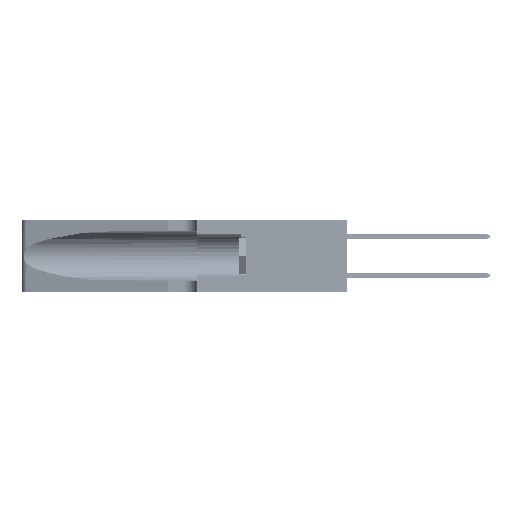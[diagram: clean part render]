
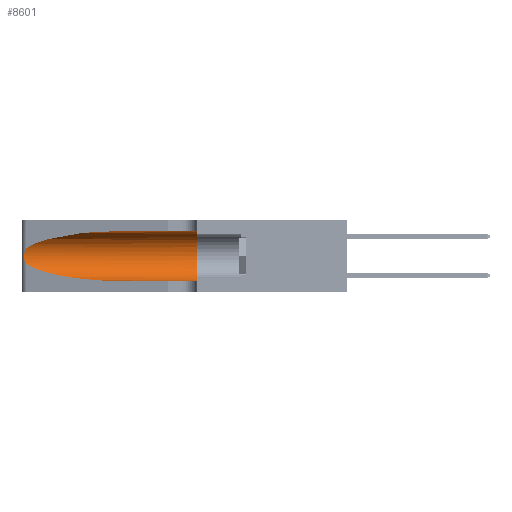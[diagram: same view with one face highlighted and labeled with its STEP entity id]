
A CAD part, left-side view. The second image highlights one B-rep face of the part: STEP entity #8601.
In plain terms, the highlighted cylindrical face has radius 3.308 mm (diameter 6.617 mm), a partial arc.
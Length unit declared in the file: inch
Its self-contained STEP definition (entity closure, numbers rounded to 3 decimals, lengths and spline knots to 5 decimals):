
#167 = CARTESIAN_POINT ( 'NONE',  ( 0.25555, 1.22993, 0.14849 ) ) ;
#2249 = CARTESIAN_POINT ( 'NONE',  ( 0.18966, 0.96281, 0.05475 ) ) ;
#3695 = VERTEX_POINT ( 'NONE', #17167 ) ;
#3905 = CARTESIAN_POINT ( 'NONE',  ( 0.25854, 1.2359, 0.20912 ) ) ;
#4080 = CARTESIAN_POINT ( 'NONE',  ( 0.25639, 1.23186, 0.15144 ) ) ;
#4301 = CARTESIAN_POINT ( 'NONE',  ( 0.25487, 1.22718, 0.22369 ) ) ;
#4521 = ORIENTED_EDGE ( 'NONE', *, *, #20952, .F. ) ;
#5397 = CARTESIAN_POINT ( 'NONE',  ( 0.1305, 0.72297, 0.05475 ) ) ;
#6532 = DIRECTION ( 'NONE',  ( 0., -1., 0. ) ) ;
#7057 = CARTESIAN_POINT ( 'NONE',  ( 0.1305, 0.35, 0.05475 ) ) ;
#7823 = CARTESIAN_POINT ( 'NONE',  ( 0.25639, 1.23184, 0.21858 ) ) ;
#8007 = CARTESIAN_POINT ( 'NONE',  ( 0.25555, 1.22994, 0.2215 ) ) ;
#8189 = CARTESIAN_POINT ( 'NONE',  ( 0.26017, 1.23833, 0.17102 ) ) ;
#8601 = ADVANCED_FACE ( 'NONE', ( #46828 ), #8744, .F. ) ;
#8739 = CARTESIAN_POINT ( 'NONE',  ( 0.1305, 1.61858, 0.31525 ) ) ;
#8744 = CYLINDRICAL_SURFACE ( 'NONE', #28605, 0.13025 ) ;
#10106 = CARTESIAN_POINT ( 'NONE',  ( 0.2373, 1.15595, 0.08982 ) ) ;
#12100 = CARTESIAN_POINT ( 'NONE',  ( 0.26018, 1.23835, 0.19895 ) ) ;
#12261 = CARTESIAN_POINT ( 'NONE',  ( 0.25789, 1.23486, 0.15765 ) ) ;
#12452 = CARTESIAN_POINT ( 'NONE',  ( 0.25487, 1.22718, 0.22369 ) ) ;
#12844 = CARTESIAN_POINT ( 'NONE',  ( 0.1305, 0.72297, 0.31525 ) ) ;
#14236 = CIRCLE ( 'NONE', #15270, 0.13025 ) ;
#15270 = AXIS2_PLACEMENT_3D ( 'NONE', #28436, #37074, #32482 ) ;
#17167 = CARTESIAN_POINT ( 'NONE',  ( 0.1305, 0.35, 0.31525 ) ) ;
#17754 = CARTESIAN_POINT ( 'NONE',  ( 0.25487, 1.22718, 0.14631 ) ) ;
#18202 = ORIENTED_EDGE ( 'NONE', *, *, #42422, .T. ) ;
#18742 = CARTESIAN_POINT ( 'NONE',  ( 0.1305, 1.61858, 0.185 ) ) ;
#19995 = CARTESIAN_POINT ( 'NONE',  ( 0.2373, 1.15595, 0.28018 ) ) ;
#20952 = EDGE_CURVE ( 'NONE', #24636, #3695, #47883, .T. ) ;
#21928 =( BOUNDED_CURVE ( )  B_SPLINE_CURVE ( 3, ( #35428, #36314, #19995, #4301 ),
 .UNSPECIFIED., .F., .F. ) 
 B_SPLINE_CURVE_WITH_KNOTS ( ( 4, 4 ),
 ( 1.5708, 2.84003 ),
 .UNSPECIFIED. ) 
 CURVE ( )  GEOMETRIC_REPRESENTATION_ITEM ( )  RATIONAL_B_SPLINE_CURVE ( ( 1., 0.87, 0.87, 1. ) ) 
 REPRESENTATION_ITEM ( '' )  );
#23005 = DIRECTION ( 'NONE',  ( 0., 0., -1. ) ) ;
#23527 = EDGE_CURVE ( 'NONE', #28503, #27170, #32978, .T. ) ;
#23862 = CARTESIAN_POINT ( 'NONE',  ( 0.26075, 1.23896, 0.178 ) ) ;
#24636 = VERTEX_POINT ( 'NONE', #12844 ) ;
#24721 = EDGE_LOOP ( 'NONE', ( #30583, #18202, #42601, #42850, #50619, #4521 ) ) ;
#26377 = VECTOR ( 'NONE', #6532, 39.37008 ) ;
#27170 = VERTEX_POINT ( 'NONE', #5397 ) ;
#28436 = CARTESIAN_POINT ( 'NONE',  ( 0.1305, 0.35, 0.185 ) ) ;
#28494 = CARTESIAN_POINT ( 'NONE',  ( 0.26075, 1.23896, 0.19203 ) ) ;
#28503 = VERTEX_POINT ( 'NONE', #17754 ) ;
#28605 = AXIS2_PLACEMENT_3D ( 'NONE', #18742, #30623, #23005 ) ;
#29101 = B_SPLINE_CURVE_WITH_KNOTS ( 'NONE', 3,
 ( #12452, #8007, #7823, #40839, #3905, #12100, #28494, #23862, #8189, #44564, #12261, #4080, #167, #32545 ),
 .UNSPECIFIED., .F., .F.,
 ( 4, 2, 2, 2, 2, 2, 4 ),
 ( 0., 0.00027, 0.00053, 0.00107, 0.0016, 0.00187, 0.00214 ),
 .UNSPECIFIED. ) ;
#30381 = CARTESIAN_POINT ( 'NONE',  ( 0.1305, 1.61858, 0.05475 ) ) ;
#30583 = ORIENTED_EDGE ( 'NONE', *, *, #31742, .T. ) ;
#30623 = DIRECTION ( 'NONE',  ( 0., -1., 0. ) ) ;
#31742 = EDGE_CURVE ( 'NONE', #24636, #44279, #21928, .T. ) ;
#32482 = DIRECTION ( 'NONE',  ( 0., 0., 1. ) ) ;
#32545 = CARTESIAN_POINT ( 'NONE',  ( 0.25487, 1.22718, 0.14631 ) ) ;
#32978 =( BOUNDED_CURVE ( )  B_SPLINE_CURVE ( 3, ( #37999, #10106, #2249, #46829 ),
 .UNSPECIFIED., .F., .F. ) 
 B_SPLINE_CURVE_WITH_KNOTS ( ( 4, 4 ),
 ( 3.44316, 4.71239 ),
 .UNSPECIFIED. ) 
 CURVE ( )  GEOMETRIC_REPRESENTATION_ITEM ( )  RATIONAL_B_SPLINE_CURVE ( ( 1., 0.87, 0.87, 1. ) ) 
 REPRESENTATION_ITEM ( '' )  );
#33051 = EDGE_CURVE ( 'NONE', #27170, #43038, #39670, .T. ) ;
#35428 = CARTESIAN_POINT ( 'NONE',  ( 0.1305, 0.72297, 0.31525 ) ) ;
#36314 = CARTESIAN_POINT ( 'NONE',  ( 0.18966, 0.96281, 0.31525 ) ) ;
#37074 = DIRECTION ( 'NONE',  ( 0., 1., 0. ) ) ;
#37999 = CARTESIAN_POINT ( 'NONE',  ( 0.25487, 1.22718, 0.14631 ) ) ;
#38366 = VECTOR ( 'NONE', #50125, 39.37008 ) ;
#39670 = LINE ( 'NONE', #30381, #26377 ) ;
#40839 = CARTESIAN_POINT ( 'NONE',  ( 0.25787, 1.23484, 0.2124 ) ) ;
#42422 = EDGE_CURVE ( 'NONE', #44279, #28503, #29101, .T. ) ;
#42601 = ORIENTED_EDGE ( 'NONE', *, *, #23527, .T. ) ;
#42850 = ORIENTED_EDGE ( 'NONE', *, *, #33051, .T. ) ;
#43038 = VERTEX_POINT ( 'NONE', #7057 ) ;
#43107 = EDGE_CURVE ( 'NONE', #3695, #43038, #14236, .T. ) ;
#44279 = VERTEX_POINT ( 'NONE', #51365 ) ;
#44564 = CARTESIAN_POINT ( 'NONE',  ( 0.25856, 1.23593, 0.16098 ) ) ;
#46828 = FACE_OUTER_BOUND ( 'NONE', #24721, .T. ) ;
#46829 = CARTESIAN_POINT ( 'NONE',  ( 0.1305, 0.72297, 0.05475 ) ) ;
#47883 = LINE ( 'NONE', #8739, #38366 ) ;
#50125 = DIRECTION ( 'NONE',  ( 0., -1., 0. ) ) ;
#50619 = ORIENTED_EDGE ( 'NONE', *, *, #43107, .F. ) ;
#51365 = CARTESIAN_POINT ( 'NONE',  ( 0.25487, 1.22718, 0.22369 ) ) ;
